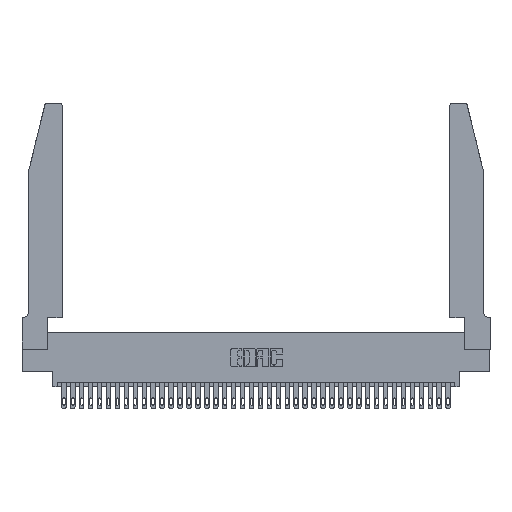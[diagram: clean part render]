
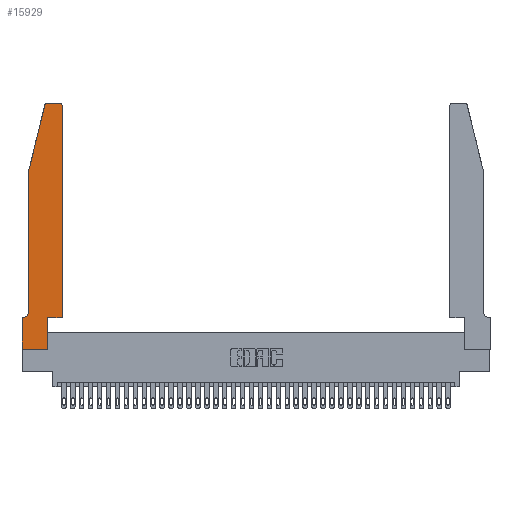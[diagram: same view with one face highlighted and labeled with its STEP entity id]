
A CAD part, top view. The second image highlights one B-rep face of the part: STEP entity #15929.
In plain terms, the highlighted planar face has unit normal (0, 0, 1).
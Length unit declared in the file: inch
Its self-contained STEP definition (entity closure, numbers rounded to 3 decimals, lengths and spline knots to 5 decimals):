
#942 = DIRECTION ( 'NONE',  ( 0., -1., 0. ) ) ;
#1603 = LINE ( 'NONE', #3599, #4469 ) ;
#2503 = CARTESIAN_POINT ( 'NONE',  ( 0., 0., 0.37 ) ) ;
#3470 = ORIENTED_EDGE ( 'NONE', *, *, #38839, .T. ) ;
#3567 = EDGE_CURVE ( 'NONE', #4831, #17062, #30690, .T. ) ;
#3599 = CARTESIAN_POINT ( 'NONE',  ( 0.4505, 0.35, 0.37 ) ) ;
#3661 = DIRECTION ( 'NONE',  ( 1., 0., 0. ) ) ;
#4469 = VECTOR ( 'NONE', #9483, 39.37008 ) ;
#4819 = VERTEX_POINT ( 'NONE', #11884 ) ;
#4831 = VERTEX_POINT ( 'NONE', #23890 ) ;
#4873 = VECTOR ( 'NONE', #6904, 39.37008 ) ;
#5903 = VECTOR ( 'NONE', #14208, 39.37008 ) ;
#5941 = CARTESIAN_POINT ( 'NONE',  ( 0.0755, 2., 0.37 ) ) ;
#6541 = ORIENTED_EDGE ( 'NONE', *, *, #24603, .T. ) ;
#6904 = DIRECTION ( 'NONE',  ( -1., 0., 0. ) ) ;
#7369 = CARTESIAN_POINT ( 'NONE',  ( 0.4205, 2.72, 0.37 ) ) ;
#7480 = EDGE_CURVE ( 'NONE', #9024, #30975, #35622, .T. ) ;
#7574 = LINE ( 'NONE', #17392, #38876 ) ;
#8090 = CARTESIAN_POINT ( 'NONE',  ( 0.284, 2.72, 0.37 ) ) ;
#8125 = CARTESIAN_POINT ( 'NONE',  ( 0.2865, 0., 0.37 ) ) ;
#9024 = VERTEX_POINT ( 'NONE', #32190 ) ;
#9304 = EDGE_CURVE ( 'NONE', #24700, #13832, #28056, .T. ) ;
#9483 = DIRECTION ( 'NONE',  ( 1., 0., 0. ) ) ;
#9765 = ORIENTED_EDGE ( 'NONE', *, *, #20905, .T. ) ;
#9871 = DIRECTION ( 'NONE',  ( -1., 0., 0. ) ) ;
#9989 = CARTESIAN_POINT ( 'NONE',  ( 0.0055, 0.42, 0.37 ) ) ;
#10260 = DIRECTION ( 'NONE',  ( 1., 0., 0. ) ) ;
#11884 = CARTESIAN_POINT ( 'NONE',  ( 0., 0.35, 0.37 ) ) ;
#13171 = VECTOR ( 'NONE', #32032, 39.37008 ) ;
#13512 = ORIENTED_EDGE ( 'NONE', *, *, #25811, .T. ) ;
#13587 = DIRECTION ( 'NONE',  ( -1., 0., 0. ) ) ;
#13832 = VERTEX_POINT ( 'NONE', #35507 ) ;
#13984 = CARTESIAN_POINT ( 'NONE',  ( 0.2605, 2.75, 0.37 ) ) ;
#14208 = DIRECTION ( 'NONE',  ( 0., 1., 0. ) ) ;
#14563 = CARTESIAN_POINT ( 'NONE',  ( 0.0755, 0.35, 0.37 ) ) ;
#15737 = ORIENTED_EDGE ( 'NONE', *, *, #21625, .T. ) ;
#15929 = ADVANCED_FACE ( 'NONE', ( #18051 ), #38714, .T. ) ;
#16481 = ORIENTED_EDGE ( 'NONE', *, *, #7480, .T. ) ;
#17062 = VERTEX_POINT ( 'NONE', #23600 ) ;
#17233 = DIRECTION ( 'NONE',  ( 0., 0., 1. ) ) ;
#17392 = CARTESIAN_POINT ( 'NONE',  ( 0., 0., 0.37 ) ) ;
#18051 = FACE_OUTER_BOUND ( 'NONE', #35525, .T. ) ;
#18100 = LINE ( 'NONE', #14563, #4873 ) ;
#18424 = VERTEX_POINT ( 'NONE', #2503 ) ;
#18755 = ORIENTED_EDGE ( 'NONE', *, *, #34694, .T. ) ;
#18784 = CIRCLE ( 'NONE', #33769, 0.03 ) ;
#19028 = AXIS2_PLACEMENT_3D ( 'NONE', #8090, #17233, #35121 ) ;
#20850 = VERTEX_POINT ( 'NONE', #23053 ) ;
#20905 = EDGE_CURVE ( 'NONE', #38956, #20850, #32454, .T. ) ;
#21625 = EDGE_CURVE ( 'NONE', #30975, #4819, #18100, .T. ) ;
#22525 = CARTESIAN_POINT ( 'NONE',  ( 0., 0., 0.37 ) ) ;
#22577 = VECTOR ( 'NONE', #27245, 39.37008 ) ;
#22741 = EDGE_CURVE ( 'NONE', #25967, #22972, #23111, .T. ) ;
#22972 = VERTEX_POINT ( 'NONE', #34772 ) ;
#23047 = ORIENTED_EDGE ( 'NONE', *, *, #32488, .T. ) ;
#23053 = CARTESIAN_POINT ( 'NONE',  ( 0.2865, 0.35, 0.37 ) ) ;
#23111 = LINE ( 'NONE', #28960, #13171 ) ;
#23339 = EDGE_CURVE ( 'NONE', #22972, #24700, #18784, .T. ) ;
#23600 = CARTESIAN_POINT ( 'NONE',  ( 0.0755, 2., 0.37 ) ) ;
#23845 = ORIENTED_EDGE ( 'NONE', *, *, #23339, .T. ) ;
#23890 = CARTESIAN_POINT ( 'NONE',  ( 0.25487, 2.72718, 0.37 ) ) ;
#24085 = ORIENTED_EDGE ( 'NONE', *, *, #9304, .T. ) ;
#24388 = CARTESIAN_POINT ( 'NONE',  ( 0., 0.35, 0.37 ) ) ;
#24603 = EDGE_CURVE ( 'NONE', #13832, #4831, #31085, .T. ) ;
#24700 = VERTEX_POINT ( 'NONE', #30267 ) ;
#24949 = CARTESIAN_POINT ( 'NONE',  ( 0.0755, 2., 0.37 ) ) ;
#25811 = EDGE_CURVE ( 'NONE', #17062, #9024, #31480, .T. ) ;
#25967 = VERTEX_POINT ( 'NONE', #32749 ) ;
#27245 = DIRECTION ( 'NONE',  ( -0.239, -0.971, 0. ) ) ;
#28056 = LINE ( 'NONE', #13984, #31875 ) ;
#28937 = ORIENTED_EDGE ( 'NONE', *, *, #3567, .T. ) ;
#28960 = CARTESIAN_POINT ( 'NONE',  ( 0.4505, 0.35, 0.37 ) ) ;
#30267 = CARTESIAN_POINT ( 'NONE',  ( 0.4205, 2.75, 0.37 ) ) ;
#30599 = ORIENTED_EDGE ( 'NONE', *, *, #22741, .T. ) ;
#30690 = LINE ( 'NONE', #5941, #22577 ) ;
#30806 = AXIS2_PLACEMENT_3D ( 'NONE', #24388, #36569, #3661 ) ;
#30975 = VERTEX_POINT ( 'NONE', #35721 ) ;
#31011 = AXIS2_PLACEMENT_3D ( 'NONE', #9989, #36730, #9871 ) ;
#31085 = CIRCLE ( 'NONE', #19028, 0.03 ) ;
#31480 = LINE ( 'NONE', #24949, #35755 ) ;
#31767 = DIRECTION ( 'NONE',  ( 0., 0., 1. ) ) ;
#31875 = VECTOR ( 'NONE', #13587, 39.37008 ) ;
#32032 = DIRECTION ( 'NONE',  ( 0., 1., 0. ) ) ;
#32190 = CARTESIAN_POINT ( 'NONE',  ( 0.0755, 0.42, 0.37 ) ) ;
#32309 = DIRECTION ( 'NONE',  ( 1., 0., 0. ) ) ;
#32454 = LINE ( 'NONE', #35536, #5903 ) ;
#32488 = EDGE_CURVE ( 'NONE', #20850, #25967, #1603, .T. ) ;
#32749 = CARTESIAN_POINT ( 'NONE',  ( 0.4505, 0.35, 0.37 ) ) ;
#32952 = DIRECTION ( 'NONE',  ( 0., -1., 0. ) ) ;
#33769 = AXIS2_PLACEMENT_3D ( 'NONE', #7369, #31767, #32309 ) ;
#34694 = EDGE_CURVE ( 'NONE', #4819, #18424, #7574, .T. ) ;
#34772 = CARTESIAN_POINT ( 'NONE',  ( 0.4505, 2.72, 0.37 ) ) ;
#35121 = DIRECTION ( 'NONE',  ( 1., 0., 0. ) ) ;
#35507 = CARTESIAN_POINT ( 'NONE',  ( 0.284, 2.75, 0.37 ) ) ;
#35525 = EDGE_LOOP ( 'NONE', ( #24085, #6541, #28937, #13512, #16481, #15737, #18755, #3470, #9765, #23047, #30599, #23845 ) ) ;
#35536 = CARTESIAN_POINT ( 'NONE',  ( 0.2865, 0.35, 0.37 ) ) ;
#35622 = CIRCLE ( 'NONE', #31011, 0.07 ) ;
#35721 = CARTESIAN_POINT ( 'NONE',  ( 0.0055, 0.35, 0.37 ) ) ;
#35755 = VECTOR ( 'NONE', #942, 39.37008 ) ;
#36161 = VECTOR ( 'NONE', #10260, 39.37008 ) ;
#36569 = DIRECTION ( 'NONE',  ( 0., 0., 1. ) ) ;
#36730 = DIRECTION ( 'NONE',  ( 0., 0., -1. ) ) ;
#38458 = LINE ( 'NONE', #22525, #36161 ) ;
#38714 = PLANE ( 'NONE',  #30806 ) ;
#38839 = EDGE_CURVE ( 'NONE', #18424, #38956, #38458, .T. ) ;
#38876 = VECTOR ( 'NONE', #32952, 39.37008 ) ;
#38956 = VERTEX_POINT ( 'NONE', #8125 ) ;
